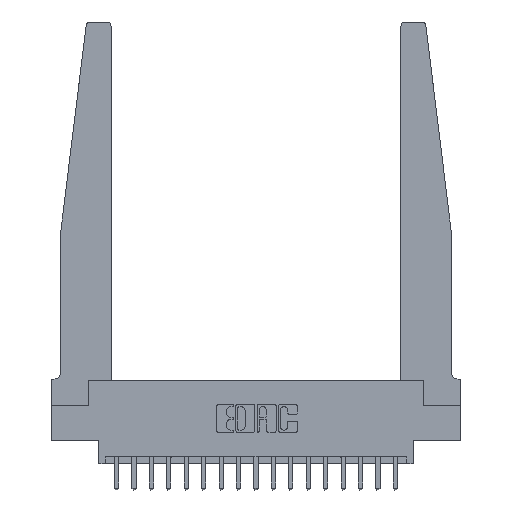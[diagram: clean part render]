
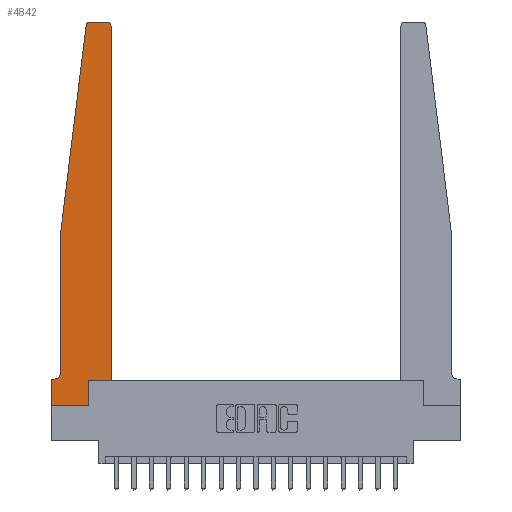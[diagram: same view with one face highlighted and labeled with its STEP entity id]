
A CAD part, top view. The second image highlights one B-rep face of the part: STEP entity #4842.
In plain terms, the highlighted planar face has unit normal (0, 0, 1).
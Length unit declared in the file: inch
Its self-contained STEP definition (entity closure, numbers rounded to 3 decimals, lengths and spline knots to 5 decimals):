
#239 = VERTEX_POINT ( 'NONE', #732 ) ;
#726 = CARTESIAN_POINT ( 'NONE',  ( 0.25, 2.75, 0.37 ) ) ;
#732 = CARTESIAN_POINT ( 'NONE',  ( 0.065, 0.2375, 0.37 ) ) ;
#815 = DIRECTION ( 'NONE',  ( -1., 0., 0. ) ) ;
#827 = EDGE_CURVE ( 'NONE', #239, #10126, #10250, .T. ) ;
#1036 = CARTESIAN_POINT ( 'NONE',  ( 0.065, 1.25, 0.37 ) ) ;
#1052 = CARTESIAN_POINT ( 'NONE',  ( 0., 0.1875, 0.37 ) ) ;
#1110 = ORIENTED_EDGE ( 'NONE', *, *, #15050, .T. ) ;
#1199 = ORIENTED_EDGE ( 'NONE', *, *, #2841, .T. ) ;
#1684 = VECTOR ( 'NONE', #4089, 39.37008 ) ;
#1742 = CARTESIAN_POINT ( 'NONE',  ( 0.425, 2.72, 0.37 ) ) ;
#1756 = VECTOR ( 'NONE', #14970, 39.37008 ) ;
#2073 = CARTESIAN_POINT ( 'NONE',  ( 0., 0., 0.37 ) ) ;
#2288 = ORIENTED_EDGE ( 'NONE', *, *, #827, .T. ) ;
#2528 = ORIENTED_EDGE ( 'NONE', *, *, #10072, .T. ) ;
#2573 = ORIENTED_EDGE ( 'NONE', *, *, #13746, .T. ) ;
#2636 = VERTEX_POINT ( 'NONE', #13085 ) ;
#2795 = CARTESIAN_POINT ( 'NONE',  ( 0.065, 1.25, 0.37 ) ) ;
#2841 = EDGE_CURVE ( 'NONE', #6812, #4976, #17119, .T. ) ;
#3706 = ORIENTED_EDGE ( 'NONE', *, *, #8077, .T. ) ;
#3741 = DIRECTION ( 'NONE',  ( 0., 0., 1. ) ) ;
#3866 = VERTEX_POINT ( 'NONE', #9723 ) ;
#4089 = DIRECTION ( 'NONE',  ( -0.122, -0.992, 0. ) ) ;
#4752 = ORIENTED_EDGE ( 'NONE', *, *, #7485, .T. ) ;
#4842 = ADVANCED_FACE ( 'NONE', ( #11784 ), #15125, .T. ) ;
#4976 = VERTEX_POINT ( 'NONE', #13916 ) ;
#5159 = ORIENTED_EDGE ( 'NONE', *, *, #10952, .T. ) ;
#5182 = EDGE_CURVE ( 'NONE', #6923, #17523, #18420, .T. ) ;
#5338 = ORIENTED_EDGE ( 'NONE', *, *, #15440, .T. ) ;
#5443 = DIRECTION ( 'NONE',  ( 0., -1., 0. ) ) ;
#5549 = CARTESIAN_POINT ( 'NONE',  ( 0., 0., 0.37 ) ) ;
#5876 = CARTESIAN_POINT ( 'NONE',  ( 0.425, 0.18, 0.37 ) ) ;
#5997 = DIRECTION ( 'NONE',  ( 0., 1., 0. ) ) ;
#6812 = VERTEX_POINT ( 'NONE', #17221 ) ;
#6923 = VERTEX_POINT ( 'NONE', #14483 ) ;
#7442 = CARTESIAN_POINT ( 'NONE',  ( 0.2605, 0.18, 0.37 ) ) ;
#7485 = EDGE_CURVE ( 'NONE', #12055, #2636, #12150, .T. ) ;
#7916 = VECTOR ( 'NONE', #11430, 39.37008 ) ;
#8022 = VERTEX_POINT ( 'NONE', #14169 ) ;
#8077 = EDGE_CURVE ( 'NONE', #2636, #3866, #9254, .T. ) ;
#8286 = CARTESIAN_POINT ( 'NONE',  ( 0.065, 1.25, 0.37 ) ) ;
#8428 = AXIS2_PLACEMENT_3D ( 'NONE', #19061, #19021, #18995 ) ;
#8598 = LINE ( 'NONE', #5876, #15653 ) ;
#8942 = DIRECTION ( 'NONE',  ( 1., 0., 0. ) ) ;
#9254 = LINE ( 'NONE', #2073, #9748 ) ;
#9497 = LINE ( 'NONE', #7442, #13098 ) ;
#9557 = AXIS2_PLACEMENT_3D ( 'NONE', #12931, #3741, #14418 ) ;
#9564 = ORIENTED_EDGE ( 'NONE', *, *, #17301, .T. ) ;
#9723 = CARTESIAN_POINT ( 'NONE',  ( 0.2605, 0., 0.37 ) ) ;
#9748 = VECTOR ( 'NONE', #11261, 39.37008 ) ;
#10072 = EDGE_CURVE ( 'NONE', #18897, #239, #17389, .T. ) ;
#10126 = VERTEX_POINT ( 'NONE', #10604 ) ;
#10250 = CIRCLE ( 'NONE', #8428, 0.05 ) ;
#10518 = DIRECTION ( 'NONE',  ( 1., 0., 0. ) ) ;
#10522 = DIRECTION ( 'NONE',  ( 0., 0., 1. ) ) ;
#10538 = CARTESIAN_POINT ( 'NONE',  ( 0.27653, 2.72, 0.37 ) ) ;
#10586 = VECTOR ( 'NONE', #10669, 39.37008 ) ;
#10604 = CARTESIAN_POINT ( 'NONE',  ( 0.015, 0.1875, 0.37 ) ) ;
#10669 = DIRECTION ( 'NONE',  ( 0., 1., 0. ) ) ;
#10693 = CARTESIAN_POINT ( 'NONE',  ( 0.425, 0.18, 0.37 ) ) ;
#10809 = CIRCLE ( 'NONE', #9557, 0.03 ) ;
#10888 = ORIENTED_EDGE ( 'NONE', *, *, #5182, .T. ) ;
#10952 = EDGE_CURVE ( 'NONE', #3866, #8022, #9497, .T. ) ;
#11261 = DIRECTION ( 'NONE',  ( 1., 0., 0. ) ) ;
#11313 = LINE ( 'NONE', #18859, #18708 ) ;
#11430 = DIRECTION ( 'NONE',  ( -1., 0., 0. ) ) ;
#11698 = VECTOR ( 'NONE', #5443, 39.37008 ) ;
#11784 = FACE_OUTER_BOUND ( 'NONE', #18613, .T. ) ;
#12055 = VERTEX_POINT ( 'NONE', #1052 ) ;
#12150 = LINE ( 'NONE', #5549, #11698 ) ;
#12931 = CARTESIAN_POINT ( 'NONE',  ( 0.395, 2.72, 0.37 ) ) ;
#13085 = CARTESIAN_POINT ( 'NONE',  ( 0., 0., 0.37 ) ) ;
#13098 = VECTOR ( 'NONE', #5997, 39.37008 ) ;
#13746 = EDGE_CURVE ( 'NONE', #10126, #12055, #11313, .T. ) ;
#13916 = CARTESIAN_POINT ( 'NONE',  ( 0.24675, 2.72367, 0.37 ) ) ;
#14169 = CARTESIAN_POINT ( 'NONE',  ( 0.2605, 0.18, 0.37 ) ) ;
#14372 = EDGE_CURVE ( 'NONE', #18797, #6812, #15941, .T. ) ;
#14418 = DIRECTION ( 'NONE',  ( 1., 0., 0. ) ) ;
#14483 = CARTESIAN_POINT ( 'NONE',  ( 0.425, 0.18, 0.37 ) ) ;
#14897 = DIRECTION ( 'NONE',  ( 1., 0., 0. ) ) ;
#14911 = DIRECTION ( 'NONE',  ( 0., 0., 1. ) ) ;
#14926 = CARTESIAN_POINT ( 'NONE',  ( 0., 0.1875, 0.37 ) ) ;
#14970 = DIRECTION ( 'NONE',  ( 0., -1., 0. ) ) ;
#15050 = EDGE_CURVE ( 'NONE', #4976, #18897, #17765, .T. ) ;
#15125 = PLANE ( 'NONE',  #18293 ) ;
#15440 = EDGE_CURVE ( 'NONE', #17523, #18797, #10809, .T. ) ;
#15653 = VECTOR ( 'NONE', #8942, 39.37008 ) ;
#15941 = LINE ( 'NONE', #726, #7916 ) ;
#16980 = CARTESIAN_POINT ( 'NONE',  ( 0.395, 2.75, 0.37 ) ) ;
#17119 = CIRCLE ( 'NONE', #17569, 0.03 ) ;
#17221 = CARTESIAN_POINT ( 'NONE',  ( 0.27653, 2.75, 0.37 ) ) ;
#17301 = EDGE_CURVE ( 'NONE', #8022, #6923, #8598, .T. ) ;
#17389 = LINE ( 'NONE', #2795, #1756 ) ;
#17523 = VERTEX_POINT ( 'NONE', #1742 ) ;
#17569 = AXIS2_PLACEMENT_3D ( 'NONE', #10538, #10522, #10518 ) ;
#17765 = LINE ( 'NONE', #1036, #1684 ) ;
#18293 = AXIS2_PLACEMENT_3D ( 'NONE', #14926, #14911, #14897 ) ;
#18420 = LINE ( 'NONE', #10693, #10586 ) ;
#18613 = EDGE_LOOP ( 'NONE', ( #18852, #1199, #1110, #2528, #2288, #2573, #4752, #3706, #5159, #9564, #10888, #5338 ) ) ;
#18708 = VECTOR ( 'NONE', #815, 39.37008 ) ;
#18797 = VERTEX_POINT ( 'NONE', #16980 ) ;
#18852 = ORIENTED_EDGE ( 'NONE', *, *, #14372, .T. ) ;
#18859 = CARTESIAN_POINT ( 'NONE',  ( 0.065, 0.1875, 0.37 ) ) ;
#18897 = VERTEX_POINT ( 'NONE', #8286 ) ;
#18995 = DIRECTION ( 'NONE',  ( -1., 0., 0. ) ) ;
#19021 = DIRECTION ( 'NONE',  ( 0., 0., -1. ) ) ;
#19061 = CARTESIAN_POINT ( 'NONE',  ( 0.015, 0.2375, 0.37 ) ) ;
